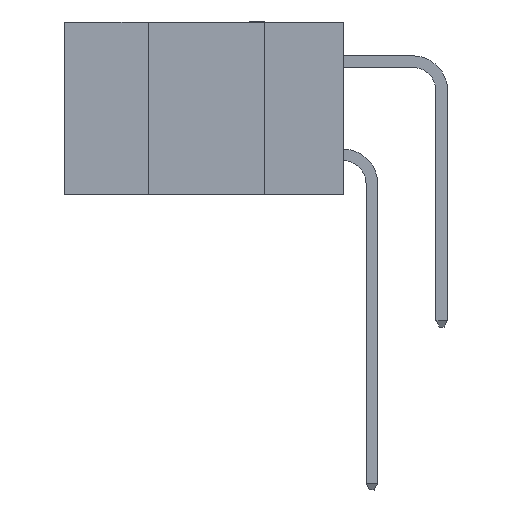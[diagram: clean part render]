
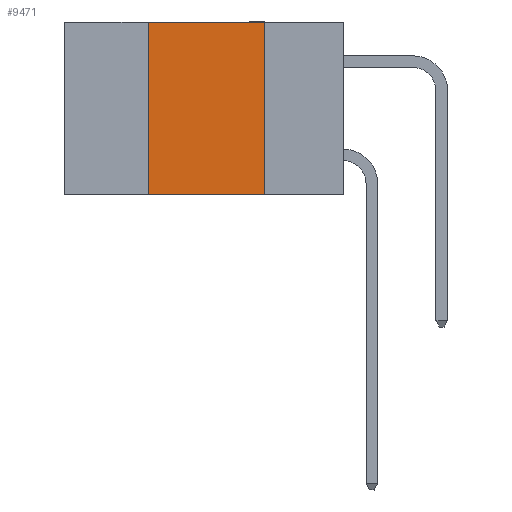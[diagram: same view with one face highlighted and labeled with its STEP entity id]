
A CAD part, left-side view. The second image highlights one B-rep face of the part: STEP entity #9471.
In plain terms, the highlighted planar face has unit normal (-1, 0, 0).
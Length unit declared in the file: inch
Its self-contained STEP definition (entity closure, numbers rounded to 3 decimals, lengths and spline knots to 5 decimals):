
#1058 = EDGE_CURVE ( 'NONE', #17967, #15541, #6987, .T. ) ;
#1492 = VECTOR ( 'NONE', #4315, 39.37008 ) ;
#1535 = CARTESIAN_POINT ( 'NONE',  ( 0., 0.6, -0.37 ) ) ;
#2805 = CARTESIAN_POINT ( 'NONE',  ( 0., 0.6, 0. ) ) ;
#2972 = VECTOR ( 'NONE', #10813, 39.37008 ) ;
#3288 = AXIS2_PLACEMENT_3D ( 'NONE', #13969, #15435, #6636 ) ;
#3439 = PLANE ( 'NONE',  #3288 ) ;
#3606 = EDGE_CURVE ( 'NONE', #4084, #17967, #5563, .T. ) ;
#4084 = VERTEX_POINT ( 'NONE', #12360 ) ;
#4129 = ORIENTED_EDGE ( 'NONE', *, *, #1058, .F. ) ;
#4315 = DIRECTION ( 'NONE',  ( 0., -1., 0. ) ) ;
#5037 = ORIENTED_EDGE ( 'NONE', *, *, #12494, .T. ) ;
#5128 = CARTESIAN_POINT ( 'NONE',  ( 0., 0.42, -0.37 ) ) ;
#5184 = EDGE_LOOP ( 'NONE', ( #4129, #5535, #18497, #5037 ) ) ;
#5535 = ORIENTED_EDGE ( 'NONE', *, *, #3606, .F. ) ;
#5563 = LINE ( 'NONE', #2805, #1492 ) ;
#6636 = DIRECTION ( 'NONE',  ( 0., 0., -1. ) ) ;
#6987 = LINE ( 'NONE', #14035, #2972 ) ;
#7327 = LINE ( 'NONE', #1535, #14698 ) ;
#7873 = DIRECTION ( 'NONE',  ( 0., 0., 1. ) ) ;
#9305 = FACE_OUTER_BOUND ( 'NONE', #5184, .T. ) ;
#9317 = CARTESIAN_POINT ( 'NONE',  ( 0., 0.42, 0. ) ) ;
#9471 = ADVANCED_FACE ( 'NONE', ( #9305 ), #3439, .F. ) ;
#10813 = DIRECTION ( 'NONE',  ( 0., 0., -1. ) ) ;
#12360 = CARTESIAN_POINT ( 'NONE',  ( 0., 0.42, 0. ) ) ;
#12494 = EDGE_CURVE ( 'NONE', #13322, #15541, #7327, .T. ) ;
#13238 = CARTESIAN_POINT ( 'NONE',  ( 0., 0.17, 0. ) ) ;
#13322 = VERTEX_POINT ( 'NONE', #5128 ) ;
#13969 = CARTESIAN_POINT ( 'NONE',  ( 0., 0.6, 0. ) ) ;
#14035 = CARTESIAN_POINT ( 'NONE',  ( 0., 0.17, 0. ) ) ;
#14412 = VECTOR ( 'NONE', #7873, 39.37008 ) ;
#14698 = VECTOR ( 'NONE', #16383, 39.37008 ) ;
#15435 = DIRECTION ( 'NONE',  ( 1., 0., 0. ) ) ;
#15541 = VERTEX_POINT ( 'NONE', #18170 ) ;
#16383 = DIRECTION ( 'NONE',  ( 0., -1., 0. ) ) ;
#17967 = VERTEX_POINT ( 'NONE', #13238 ) ;
#18169 = LINE ( 'NONE', #9317, #14412 ) ;
#18170 = CARTESIAN_POINT ( 'NONE',  ( 0., 0.17, -0.37 ) ) ;
#18208 = EDGE_CURVE ( 'NONE', #13322, #4084, #18169, .T. ) ;
#18497 = ORIENTED_EDGE ( 'NONE', *, *, #18208, .F. ) ;
